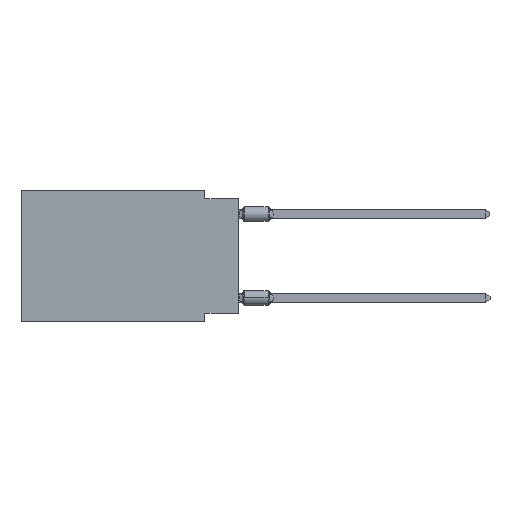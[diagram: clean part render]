
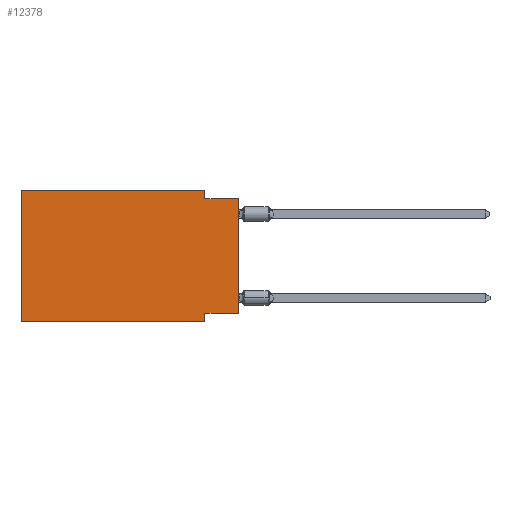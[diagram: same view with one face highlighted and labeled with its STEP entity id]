
A CAD part, left-side view. The second image highlights one B-rep face of the part: STEP entity #12378.
In plain terms, the highlighted planar face has unit normal (-1, 0, 0).
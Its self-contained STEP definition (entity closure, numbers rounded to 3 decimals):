
#384 = CARTESIAN_POINT ( 'NONE',  ( 0., 0., -9.271 ) ) ;
#394 = EDGE_CURVE ( 'NONE', #16421, #6725, #13790, .T. ) ;
#486 = CARTESIAN_POINT ( 'NONE',  ( 0., 0., -0.635 ) ) ;
#723 = CARTESIAN_POINT ( 'NONE',  ( 0., 2.54, -9.906 ) ) ;
#1457 = LINE ( 'NONE', #7609, #17787 ) ;
#1830 = DIRECTION ( 'NONE',  ( 0., -1., 0. ) ) ;
#2009 = ORIENTED_EDGE ( 'NONE', *, *, #18410, .T. ) ;
#2225 = LINE ( 'NONE', #723, #3528 ) ;
#2259 = LINE ( 'NONE', #11543, #2455 ) ;
#2455 = VECTOR ( 'NONE', #19130, 1000. ) ;
#2501 = DIRECTION ( 'NONE',  ( 1., 0., 0. ) ) ;
#3119 = DIRECTION ( 'NONE',  ( 0., 0., 1. ) ) ;
#3230 = ORIENTED_EDGE ( 'NONE', *, *, #8390, .F. ) ;
#3333 = CARTESIAN_POINT ( 'NONE',  ( 0., 0., 0. ) ) ;
#3528 = VECTOR ( 'NONE', #6864, 1000. ) ;
#3582 = CARTESIAN_POINT ( 'NONE',  ( 0., 16.383, -9.906 ) ) ;
#4076 = VECTOR ( 'NONE', #1830, 1000. ) ;
#4322 = ORIENTED_EDGE ( 'NONE', *, *, #9111, .F. ) ;
#4344 = VERTEX_POINT ( 'NONE', #12527 ) ;
#4710 = DIRECTION ( 'NONE',  ( 0., 1., 0. ) ) ;
#4748 = LINE ( 'NONE', #5412, #4076 ) ;
#4934 = LINE ( 'NONE', #3333, #18388 ) ;
#5123 = EDGE_CURVE ( 'NONE', #4344, #19880, #2225, .T. ) ;
#5393 = EDGE_LOOP ( 'NONE', ( #14020, #14205, #17720, #15871, #4322, #2009, #11780, #3230 ) ) ;
#5412 = CARTESIAN_POINT ( 'NONE',  ( 0., 0., -0.635 ) ) ;
#5619 = DIRECTION ( 'NONE',  ( 0., 0., -1. ) ) ;
#5999 = PLANE ( 'NONE',  #11444 ) ;
#6225 = LINE ( 'NONE', #384, #17669 ) ;
#6421 = EDGE_CURVE ( 'NONE', #14969, #16421, #2259, .T. ) ;
#6725 = VERTEX_POINT ( 'NONE', #15880 ) ;
#6814 = EDGE_CURVE ( 'NONE', #6725, #10924, #4748, .T. ) ;
#6831 = CARTESIAN_POINT ( 'NONE',  ( 0., 2.54, 0. ) ) ;
#6864 = DIRECTION ( 'NONE',  ( 0., 0., -1. ) ) ;
#7134 = VECTOR ( 'NONE', #18220, 1000. ) ;
#7381 = LINE ( 'NONE', #12051, #13202 ) ;
#7609 = CARTESIAN_POINT ( 'NONE',  ( 0., 16.383, -9.906 ) ) ;
#8390 = EDGE_CURVE ( 'NONE', #17414, #4344, #6225, .T. ) ;
#9111 = EDGE_CURVE ( 'NONE', #19818, #14969, #7381, .T. ) ;
#9313 = CARTESIAN_POINT ( 'NONE',  ( 0., 2.54, 0. ) ) ;
#10924 = VERTEX_POINT ( 'NONE', #486 ) ;
#11444 = AXIS2_PLACEMENT_3D ( 'NONE', #16345, #2501, #5619 ) ;
#11543 = CARTESIAN_POINT ( 'NONE',  ( 0., 16.383, 0. ) ) ;
#11780 = ORIENTED_EDGE ( 'NONE', *, *, #5123, .F. ) ;
#12051 = CARTESIAN_POINT ( 'NONE',  ( 0., 16.383, 0. ) ) ;
#12378 = ADVANCED_FACE ( 'NONE', ( #19862 ), #5999, .F. ) ;
#12527 = CARTESIAN_POINT ( 'NONE',  ( 0., 2.54, -9.271 ) ) ;
#13202 = VECTOR ( 'NONE', #18695, 1000. ) ;
#13339 = CARTESIAN_POINT ( 'NONE',  ( 0., 16.383, 0. ) ) ;
#13790 = LINE ( 'NONE', #9313, #7134 ) ;
#14020 = ORIENTED_EDGE ( 'NONE', *, *, #17561, .T. ) ;
#14205 = ORIENTED_EDGE ( 'NONE', *, *, #6814, .F. ) ;
#14969 = VERTEX_POINT ( 'NONE', #13339 ) ;
#15871 = ORIENTED_EDGE ( 'NONE', *, *, #6421, .F. ) ;
#15880 = CARTESIAN_POINT ( 'NONE',  ( 0., 2.54, -0.635 ) ) ;
#15910 = CARTESIAN_POINT ( 'NONE',  ( 0., 2.54, -9.906 ) ) ;
#16345 = CARTESIAN_POINT ( 'NONE',  ( 0., 16.383, 0. ) ) ;
#16421 = VERTEX_POINT ( 'NONE', #6831 ) ;
#16490 = CARTESIAN_POINT ( 'NONE',  ( 0., 0., -9.271 ) ) ;
#17414 = VERTEX_POINT ( 'NONE', #16490 ) ;
#17561 = EDGE_CURVE ( 'NONE', #17414, #10924, #4934, .T. ) ;
#17669 = VECTOR ( 'NONE', #4710, 1000. ) ;
#17720 = ORIENTED_EDGE ( 'NONE', *, *, #394, .F. ) ;
#17787 = VECTOR ( 'NONE', #19846, 1000. ) ;
#18220 = DIRECTION ( 'NONE',  ( 0., 0., -1. ) ) ;
#18388 = VECTOR ( 'NONE', #3119, 1000. ) ;
#18410 = EDGE_CURVE ( 'NONE', #19818, #19880, #1457, .T. ) ;
#18695 = DIRECTION ( 'NONE',  ( 0., 0., 1. ) ) ;
#19130 = DIRECTION ( 'NONE',  ( 0., -1., 0. ) ) ;
#19818 = VERTEX_POINT ( 'NONE', #3582 ) ;
#19846 = DIRECTION ( 'NONE',  ( 0., -1., 0. ) ) ;
#19862 = FACE_OUTER_BOUND ( 'NONE', #5393, .T. ) ;
#19880 = VERTEX_POINT ( 'NONE', #15910 ) ;
